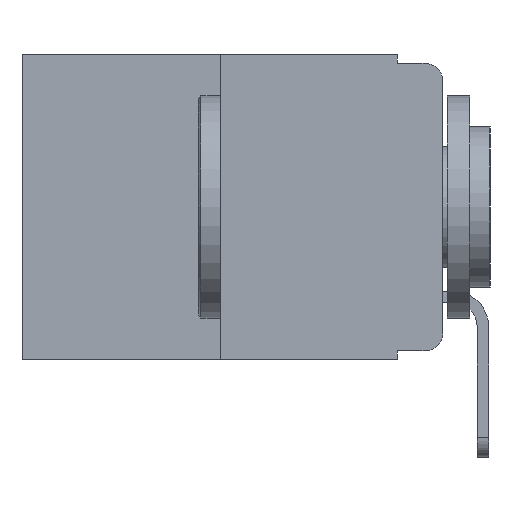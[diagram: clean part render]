
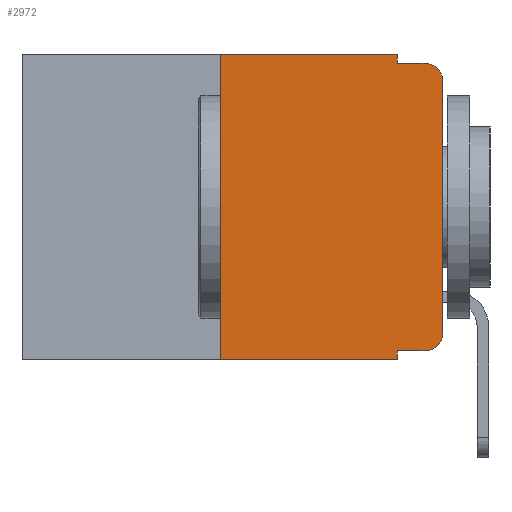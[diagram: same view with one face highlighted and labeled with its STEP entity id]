
A CAD part, left-side view. The second image highlights one B-rep face of the part: STEP entity #2972.
In plain terms, the highlighted planar face has unit normal (-1, 0, 0).
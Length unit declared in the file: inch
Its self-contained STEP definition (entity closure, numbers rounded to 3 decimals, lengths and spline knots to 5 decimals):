
#81 = LINE ( 'NONE', #2332, #1362 ) ;
#134 = VECTOR ( 'NONE', #12785, 39.37008 ) ;
#182 = CARTESIAN_POINT ( 'NONE',  ( 0., 0.02, -0.333 ) ) ;
#195 = CIRCLE ( 'NONE', #3661, 0.02 ) ;
#407 = CARTESIAN_POINT ( 'NONE',  ( 0., 0.051, -0.01 ) ) ;
#502 = CARTESIAN_POINT ( 'NONE',  ( 0., 0.02, -0.03 ) ) ;
#521 = ORIENTED_EDGE ( 'NONE', *, *, #14680, .F. ) ;
#751 = VERTEX_POINT ( 'NONE', #6819 ) ;
#1285 = VERTEX_POINT ( 'NONE', #13855 ) ;
#1309 = LINE ( 'NONE', #4890, #134 ) ;
#1362 = VECTOR ( 'NONE', #13848, 39.37008 ) ;
#1676 = AXIS2_PLACEMENT_3D ( 'NONE', #14130, #9414, #8169 ) ;
#1731 = EDGE_CURVE ( 'NONE', #8232, #6554, #9257, .T. ) ;
#2105 = VECTOR ( 'NONE', #5139, 39.37008 ) ;
#2230 = LINE ( 'NONE', #6942, #14874 ) ;
#2332 = CARTESIAN_POINT ( 'NONE',  ( 0., 0.473, 0. ) ) ;
#2473 = VERTEX_POINT ( 'NONE', #6468 ) ;
#2503 = ORIENTED_EDGE ( 'NONE', *, *, #10433, .T. ) ;
#2517 = VECTOR ( 'NONE', #5213, 39.37008 ) ;
#2617 = CARTESIAN_POINT ( 'NONE',  ( 0., 0.051, 0. ) ) ;
#2776 = VECTOR ( 'NONE', #13684, 39.37008 ) ;
#2828 = ORIENTED_EDGE ( 'NONE', *, *, #7401, .T. ) ;
#2972 = ADVANCED_FACE ( 'NONE', ( #11195 ), #13763, .F. ) ;
#3031 = LINE ( 'NONE', #407, #2517 ) ;
#3109 = CARTESIAN_POINT ( 'NONE',  ( 0., 0.473, 0. ) ) ;
#3572 = EDGE_CURVE ( 'NONE', #751, #8586, #3031, .T. ) ;
#3661 = AXIS2_PLACEMENT_3D ( 'NONE', #502, #12194, #9921 ) ;
#3847 = ORIENTED_EDGE ( 'NONE', *, *, #10676, .F. ) ;
#4326 = CARTESIAN_POINT ( 'NONE',  ( 0., 0.051, -0.333 ) ) ;
#4634 = DIRECTION ( 'NONE',  ( 0., 0., 1. ) ) ;
#4890 = CARTESIAN_POINT ( 'NONE',  ( 0., 0.051, 0. ) ) ;
#4972 = EDGE_CURVE ( 'NONE', #8643, #8860, #13181, .T. ) ;
#5139 = DIRECTION ( 'NONE',  ( 0., 0., 1. ) ) ;
#5213 = DIRECTION ( 'NONE',  ( 0., -1., 0. ) ) ;
#5221 = LINE ( 'NONE', #7288, #2105 ) ;
#5437 = VERTEX_POINT ( 'NONE', #13929 ) ;
#5600 = VERTEX_POINT ( 'NONE', #9885 ) ;
#5759 = CARTESIAN_POINT ( 'NONE',  ( 0., 0.051, -0.343 ) ) ;
#6468 = CARTESIAN_POINT ( 'NONE',  ( 0., 0.051, 0. ) ) ;
#6554 = VERTEX_POINT ( 'NONE', #182 ) ;
#6591 = EDGE_CURVE ( 'NONE', #8643, #5437, #2230, .T. ) ;
#6819 = CARTESIAN_POINT ( 'NONE',  ( 0., 0.051, -0.01 ) ) ;
#6942 = CARTESIAN_POINT ( 'NONE',  ( 0., 0.25, 0. ) ) ;
#7288 = CARTESIAN_POINT ( 'NONE',  ( 0., 0., 0. ) ) ;
#7383 = DIRECTION ( 'NONE',  ( 0., -1., 0. ) ) ;
#7401 = EDGE_CURVE ( 'NONE', #1285, #8586, #195, .T. ) ;
#7734 = ORIENTED_EDGE ( 'NONE', *, *, #3572, .F. ) ;
#7849 = CARTESIAN_POINT ( 'NONE',  ( 0., 0.25, -0.343 ) ) ;
#7872 = CARTESIAN_POINT ( 'NONE',  ( 0., 0.051, -0.333 ) ) ;
#8169 = DIRECTION ( 'NONE',  ( 0., 0., -1. ) ) ;
#8171 = ORIENTED_EDGE ( 'NONE', *, *, #10633, .F. ) ;
#8232 = VERTEX_POINT ( 'NONE', #7872 ) ;
#8404 = LINE ( 'NONE', #2617, #11759 ) ;
#8586 = VERTEX_POINT ( 'NONE', #8684 ) ;
#8643 = VERTEX_POINT ( 'NONE', #7849 ) ;
#8684 = CARTESIAN_POINT ( 'NONE',  ( 0., 0.02, -0.01 ) ) ;
#8860 = VERTEX_POINT ( 'NONE', #5759 ) ;
#9231 = ORIENTED_EDGE ( 'NONE', *, *, #6591, .F. ) ;
#9257 = LINE ( 'NONE', #4326, #2776 ) ;
#9414 = DIRECTION ( 'NONE',  ( -1., 0., 0. ) ) ;
#9684 = ORIENTED_EDGE ( 'NONE', *, *, #14685, .T. ) ;
#9885 = CARTESIAN_POINT ( 'NONE',  ( 0., 0., -0.313 ) ) ;
#9921 = DIRECTION ( 'NONE',  ( 0., 0., -1. ) ) ;
#10433 = EDGE_CURVE ( 'NONE', #5600, #1285, #5221, .T. ) ;
#10633 = EDGE_CURVE ( 'NONE', #8232, #8860, #1309, .T. ) ;
#10676 = EDGE_CURVE ( 'NONE', #5437, #2473, #81, .T. ) ;
#11195 = FACE_OUTER_BOUND ( 'NONE', #11892, .T. ) ;
#11349 = DIRECTION ( 'NONE',  ( 0., 0., -1. ) ) ;
#11606 = ORIENTED_EDGE ( 'NONE', *, *, #4972, .T. ) ;
#11759 = VECTOR ( 'NONE', #11925, 39.37008 ) ;
#11892 = EDGE_LOOP ( 'NONE', ( #2503, #2828, #7734, #521, #3847, #9231, #11606, #8171, #11906, #9684 ) ) ;
#11906 = ORIENTED_EDGE ( 'NONE', *, *, #1731, .T. ) ;
#11925 = DIRECTION ( 'NONE',  ( 0., 0., -1. ) ) ;
#12194 = DIRECTION ( 'NONE',  ( -1., 0., 0. ) ) ;
#12785 = DIRECTION ( 'NONE',  ( 0., 0., -1. ) ) ;
#13181 = LINE ( 'NONE', #14559, #14573 ) ;
#13527 = DIRECTION ( 'NONE',  ( 1., 0., 0. ) ) ;
#13684 = DIRECTION ( 'NONE',  ( 0., -1., 0. ) ) ;
#13763 = PLANE ( 'NONE',  #14753 ) ;
#13848 = DIRECTION ( 'NONE',  ( 0., -1., 0. ) ) ;
#13855 = CARTESIAN_POINT ( 'NONE',  ( 0., 0., -0.03 ) ) ;
#13929 = CARTESIAN_POINT ( 'NONE',  ( 0., 0.25, 0. ) ) ;
#14130 = CARTESIAN_POINT ( 'NONE',  ( 0., 0.02, -0.313 ) ) ;
#14559 = CARTESIAN_POINT ( 'NONE',  ( 0., 0.473, -0.343 ) ) ;
#14573 = VECTOR ( 'NONE', #7383, 39.37008 ) ;
#14680 = EDGE_CURVE ( 'NONE', #2473, #751, #8404, .T. ) ;
#14685 = EDGE_CURVE ( 'NONE', #6554, #5600, #14918, .T. ) ;
#14753 = AXIS2_PLACEMENT_3D ( 'NONE', #3109, #13527, #11349 ) ;
#14874 = VECTOR ( 'NONE', #4634, 39.37008 ) ;
#14918 = CIRCLE ( 'NONE', #1676, 0.02 ) ;
